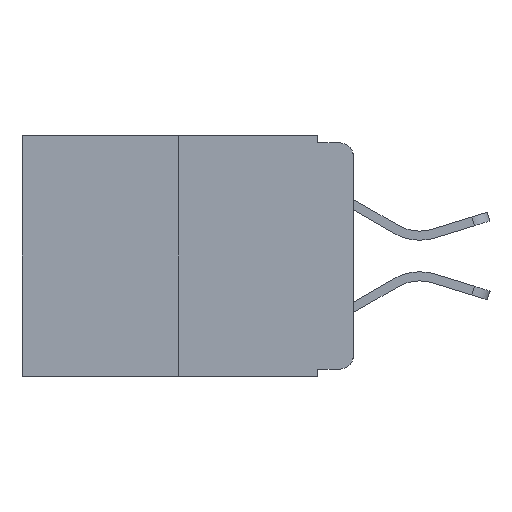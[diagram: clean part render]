
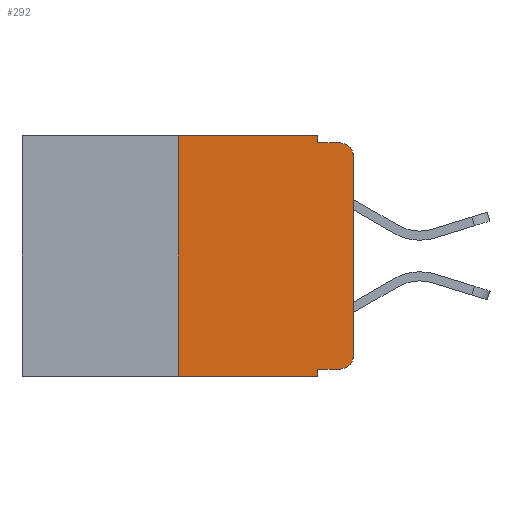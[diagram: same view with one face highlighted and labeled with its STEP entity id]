
A CAD part, left-side view. The second image highlights one B-rep face of the part: STEP entity #292.
In plain terms, the highlighted planar face has unit normal (-1, 0, 0).
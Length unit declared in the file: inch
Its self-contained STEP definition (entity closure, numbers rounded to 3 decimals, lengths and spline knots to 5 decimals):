
#40 = VERTEX_POINT ( 'NONE', #4407 ) ;
#215 = DIRECTION ( 'NONE',  ( -1., 0., 0. ) ) ;
#292 = ADVANCED_FACE ( 'NONE', ( #13966 ), #9698, .F. ) ;
#558 = AXIS2_PLACEMENT_3D ( 'NONE', #10920, #15561, #3732 ) ;
#1106 = CARTESIAN_POINT ( 'NONE',  ( 0., 0.25, 0. ) ) ;
#1135 = CARTESIAN_POINT ( 'NONE',  ( 0., 0.473, -0.343 ) ) ;
#1153 = LINE ( 'NONE', #3806, #1168 ) ;
#1168 = VECTOR ( 'NONE', #18601, 39.37008 ) ;
#1179 = EDGE_CURVE ( 'NONE', #7703, #40, #18278, .T. ) ;
#1746 = DIRECTION ( 'NONE',  ( 0., 0., -1. ) ) ;
#1858 = VECTOR ( 'NONE', #15516, 39.37008 ) ;
#2412 = CARTESIAN_POINT ( 'NONE',  ( 0., 0.051, -0.01 ) ) ;
#2732 = VERTEX_POINT ( 'NONE', #11124 ) ;
#3009 = LINE ( 'NONE', #1106, #14810 ) ;
#3732 = DIRECTION ( 'NONE',  ( 0., 0., -1. ) ) ;
#3806 = CARTESIAN_POINT ( 'NONE',  ( 0., 0., 0. ) ) ;
#3810 = VECTOR ( 'NONE', #17038, 39.37008 ) ;
#3842 = DIRECTION ( 'NONE',  ( 0., 0., -1. ) ) ;
#3931 = LINE ( 'NONE', #6858, #16158 ) ;
#4407 = CARTESIAN_POINT ( 'NONE',  ( 0., 0.02, -0.333 ) ) ;
#4486 = ORIENTED_EDGE ( 'NONE', *, *, #7187, .T. ) ;
#4729 = EDGE_CURVE ( 'NONE', #10506, #18564, #17415, .T. ) ;
#4967 = EDGE_CURVE ( 'NONE', #5146, #15492, #7557, .T. ) ;
#5146 = VERTEX_POINT ( 'NONE', #15134 ) ;
#5286 = ORIENTED_EDGE ( 'NONE', *, *, #7592, .F. ) ;
#5304 = LINE ( 'NONE', #1135, #3810 ) ;
#5698 = ORIENTED_EDGE ( 'NONE', *, *, #16090, .F. ) ;
#5718 = EDGE_CURVE ( 'NONE', #15492, #18564, #3931, .T. ) ;
#6124 = CARTESIAN_POINT ( 'NONE',  ( 0., 0.051, 0. ) ) ;
#6638 = CARTESIAN_POINT ( 'NONE',  ( 0., 0.02, -0.313 ) ) ;
#6858 = CARTESIAN_POINT ( 'NONE',  ( 0., 0.051, -0.01 ) ) ;
#7187 = EDGE_CURVE ( 'NONE', #10240, #10551, #5304, .T. ) ;
#7403 = CARTESIAN_POINT ( 'NONE',  ( 0., 0.02, -0.03 ) ) ;
#7557 = LINE ( 'NONE', #6124, #17744 ) ;
#7592 = EDGE_CURVE ( 'NONE', #7703, #10551, #15677, .T. ) ;
#7621 = DIRECTION ( 'NONE',  ( 0., -1., 0. ) ) ;
#7703 = VERTEX_POINT ( 'NONE', #17374 ) ;
#7892 = CARTESIAN_POINT ( 'NONE',  ( 0., 0., -0.03 ) ) ;
#7906 = ORIENTED_EDGE ( 'NONE', *, *, #5718, .F. ) ;
#8148 = DIRECTION ( 'NONE',  ( 0., 0., -1. ) ) ;
#8176 = ORIENTED_EDGE ( 'NONE', *, *, #15430, .T. ) ;
#8322 = ORIENTED_EDGE ( 'NONE', *, *, #4967, .F. ) ;
#9238 = AXIS2_PLACEMENT_3D ( 'NONE', #7403, #215, #1746 ) ;
#9468 = DIRECTION ( 'NONE',  ( -1., 0., 0. ) ) ;
#9656 = EDGE_CURVE ( 'NONE', #40, #2732, #11038, .T. ) ;
#9698 = PLANE ( 'NONE',  #558 ) ;
#10240 = VERTEX_POINT ( 'NONE', #12548 ) ;
#10447 = CARTESIAN_POINT ( 'NONE',  ( 0., 0.051, -0.343 ) ) ;
#10506 = VERTEX_POINT ( 'NONE', #7892 ) ;
#10551 = VERTEX_POINT ( 'NONE', #10447 ) ;
#10673 = ORIENTED_EDGE ( 'NONE', *, *, #9656, .T. ) ;
#10920 = CARTESIAN_POINT ( 'NONE',  ( 0., 0.473, 0. ) ) ;
#11038 = CIRCLE ( 'NONE', #11642, 0.02 ) ;
#11057 = CARTESIAN_POINT ( 'NONE',  ( 0., 0.051, -0.333 ) ) ;
#11124 = CARTESIAN_POINT ( 'NONE',  ( 0., 0., -0.313 ) ) ;
#11168 = EDGE_LOOP ( 'NONE', ( #8176, #13161, #7906, #8322, #5698, #17485, #4486, #5286, #17556, #10673 ) ) ;
#11202 = DIRECTION ( 'NONE',  ( 0., -1., 0. ) ) ;
#11613 = CARTESIAN_POINT ( 'NONE',  ( 0., 0.25, 0. ) ) ;
#11642 = AXIS2_PLACEMENT_3D ( 'NONE', #6638, #9468, #8148 ) ;
#12548 = CARTESIAN_POINT ( 'NONE',  ( 0., 0.25, -0.343 ) ) ;
#12809 = VECTOR ( 'NONE', #3842, 39.37008 ) ;
#13124 = CARTESIAN_POINT ( 'NONE',  ( 0., 0.473, 0. ) ) ;
#13161 = ORIENTED_EDGE ( 'NONE', *, *, #4729, .T. ) ;
#13422 = DIRECTION ( 'NONE',  ( 0., 0., -1. ) ) ;
#13501 = LINE ( 'NONE', #13124, #15422 ) ;
#13966 = FACE_OUTER_BOUND ( 'NONE', #11168, .T. ) ;
#14194 = VERTEX_POINT ( 'NONE', #11613 ) ;
#14810 = VECTOR ( 'NONE', #16354, 39.37008 ) ;
#15134 = CARTESIAN_POINT ( 'NONE',  ( 0., 0.051, 0. ) ) ;
#15422 = VECTOR ( 'NONE', #7621, 39.37008 ) ;
#15430 = EDGE_CURVE ( 'NONE', #2732, #10506, #1153, .T. ) ;
#15492 = VERTEX_POINT ( 'NONE', #2412 ) ;
#15516 = DIRECTION ( 'NONE',  ( 0., -1., 0. ) ) ;
#15561 = DIRECTION ( 'NONE',  ( 1., 0., 0. ) ) ;
#15677 = LINE ( 'NONE', #16813, #12809 ) ;
#16048 = EDGE_CURVE ( 'NONE', #10240, #14194, #3009, .T. ) ;
#16090 = EDGE_CURVE ( 'NONE', #14194, #5146, #13501, .T. ) ;
#16158 = VECTOR ( 'NONE', #11202, 39.37008 ) ;
#16354 = DIRECTION ( 'NONE',  ( 0., 0., 1. ) ) ;
#16813 = CARTESIAN_POINT ( 'NONE',  ( 0., 0.051, 0. ) ) ;
#17038 = DIRECTION ( 'NONE',  ( 0., -1., 0. ) ) ;
#17374 = CARTESIAN_POINT ( 'NONE',  ( 0., 0.051, -0.333 ) ) ;
#17415 = CIRCLE ( 'NONE', #9238, 0.02 ) ;
#17485 = ORIENTED_EDGE ( 'NONE', *, *, #16048, .F. ) ;
#17556 = ORIENTED_EDGE ( 'NONE', *, *, #1179, .T. ) ;
#17645 = CARTESIAN_POINT ( 'NONE',  ( 0., 0.02, -0.01 ) ) ;
#17744 = VECTOR ( 'NONE', #13422, 39.37008 ) ;
#18278 = LINE ( 'NONE', #11057, #1858 ) ;
#18564 = VERTEX_POINT ( 'NONE', #17645 ) ;
#18601 = DIRECTION ( 'NONE',  ( 0., 0., 1. ) ) ;
